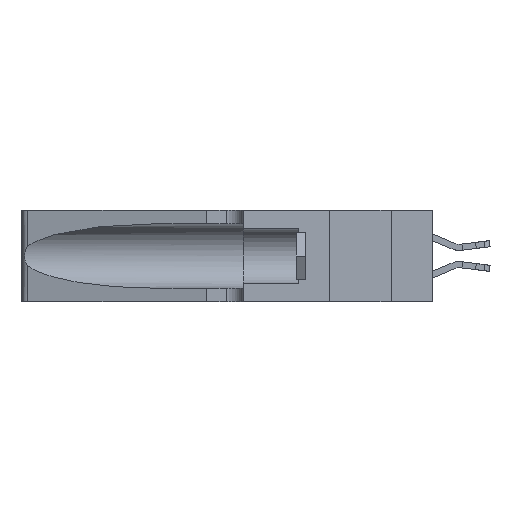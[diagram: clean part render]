
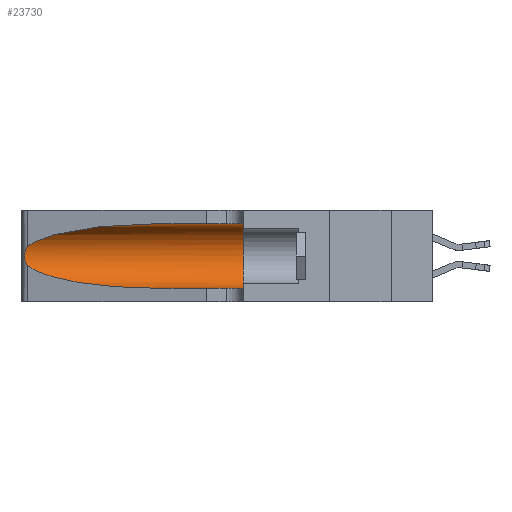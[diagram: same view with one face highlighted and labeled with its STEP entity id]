
A CAD part, left-side view. The second image highlights one B-rep face of the part: STEP entity #23730.
In plain terms, the highlighted cylindrical face has radius 3.308 mm (diameter 6.617 mm), a partial arc.
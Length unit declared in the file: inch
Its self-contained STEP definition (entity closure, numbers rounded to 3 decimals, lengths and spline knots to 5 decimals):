
#177 = DIRECTION ( 'NONE',  ( 0., -1., 0. ) ) ;
#205 = CARTESIAN_POINT ( 'NONE',  ( 0.2373, 1.15595, 0.28018 ) ) ;
#1147 = ORIENTED_EDGE ( 'NONE', *, *, #32298, .T. ) ;
#2047 = CARTESIAN_POINT ( 'NONE',  ( 0.25856, 1.23593, 0.16098 ) ) ;
#2489 = DIRECTION ( 'NONE',  ( 0., -1., 0. ) ) ;
#3336 = ORIENTED_EDGE ( 'NONE', *, *, #33354, .F. ) ;
#4023 = LINE ( 'NONE', #35388, #10461 ) ;
#4152 = DIRECTION ( 'NONE',  ( 0., -1., 0. ) ) ;
#4874 = CARTESIAN_POINT ( 'NONE',  ( 0.25639, 1.23186, 0.15144 ) ) ;
#5517 = CIRCLE ( 'NONE', #25784, 0.13025 ) ;
#5779 = EDGE_CURVE ( 'NONE', #12268, #11957, #31395, .T. ) ;
#5876 = VERTEX_POINT ( 'NONE', #25345 ) ;
#5976 = CARTESIAN_POINT ( 'NONE',  ( 0.1305, 0.72297, 0.05475 ) ) ;
#6512 = EDGE_LOOP ( 'NONE', ( #1147, #16391, #9265, #7586, #3336, #28582 ) ) ;
#6934 = CARTESIAN_POINT ( 'NONE',  ( 0.1305, 1.61858, 0.185 ) ) ;
#7407 = CARTESIAN_POINT ( 'NONE',  ( 0.25487, 1.22718, 0.22369 ) ) ;
#7586 = ORIENTED_EDGE ( 'NONE', *, *, #15427, .T. ) ;
#7638 = CARTESIAN_POINT ( 'NONE',  ( 0.25487, 1.22718, 0.14631 ) ) ;
#8464 = CARTESIAN_POINT ( 'NONE',  ( 0.25487, 1.22718, 0.14631 ) ) ;
#9265 = ORIENTED_EDGE ( 'NONE', *, *, #5779, .T. ) ;
#9838 = VERTEX_POINT ( 'NONE', #24426 ) ;
#10275 = CARTESIAN_POINT ( 'NONE',  ( 0.25639, 1.23184, 0.21858 ) ) ;
#10416 = AXIS2_PLACEMENT_3D ( 'NONE', #6934, #4152, #23348 ) ;
#10423 = DIRECTION ( 'NONE',  ( 0., 1., 0. ) ) ;
#10461 = VECTOR ( 'NONE', #2489, 39.37008 ) ;
#11229 = CARTESIAN_POINT ( 'NONE',  ( 0.18966, 0.96281, 0.31525 ) ) ;
#11402 = CARTESIAN_POINT ( 'NONE',  ( 0.25487, 1.22718, 0.22369 ) ) ;
#11957 = VERTEX_POINT ( 'NONE', #5976 ) ;
#12268 = VERTEX_POINT ( 'NONE', #29209 ) ;
#13074 = CARTESIAN_POINT ( 'NONE',  ( 0.25854, 1.2359, 0.20912 ) ) ;
#13637 = EDGE_CURVE ( 'NONE', #9838, #5876, #19664, .T. ) ;
#15140 = CARTESIAN_POINT ( 'NONE',  ( 0.1305, 0.35, 0.05475 ) ) ;
#15427 = EDGE_CURVE ( 'NONE', #11957, #34701, #4023, .T. ) ;
#15838 = CARTESIAN_POINT ( 'NONE',  ( 0.26075, 1.23896, 0.19203 ) ) ;
#16391 = ORIENTED_EDGE ( 'NONE', *, *, #26355, .T. ) ;
#16588 = VERTEX_POINT ( 'NONE', #11402 ) ;
#18579 = CARTESIAN_POINT ( 'NONE',  ( 0.26017, 1.23833, 0.17102 ) ) ;
#19403 = CARTESIAN_POINT ( 'NONE',  ( 0.18966, 0.96281, 0.05475 ) ) ;
#19521 = CARTESIAN_POINT ( 'NONE',  ( 0.25487, 1.22718, 0.22369 ) ) ;
#19664 = LINE ( 'NONE', #33135, #32472 ) ;
#21328 = CARTESIAN_POINT ( 'NONE',  ( 0.25789, 1.23486, 0.15765 ) ) ;
#22133 = CARTESIAN_POINT ( 'NONE',  ( 0.2373, 1.15595, 0.08982 ) ) ;
#23348 = DIRECTION ( 'NONE',  ( 0., 0., -1. ) ) ;
#23453 =( BOUNDED_CURVE ( )  B_SPLINE_CURVE ( 3, ( #30400, #11229, #205, #19521 ),
 .UNSPECIFIED., .F., .F. ) 
 B_SPLINE_CURVE_WITH_KNOTS ( ( 4, 4 ),
 ( 1.5708, 2.84003 ),
 .UNSPECIFIED. ) 
 CURVE ( )  GEOMETRIC_REPRESENTATION_ITEM ( )  RATIONAL_B_SPLINE_CURVE ( ( 1., 0.87, 0.87, 1. ) ) 
 REPRESENTATION_ITEM ( '' )  );
#23730 = ADVANCED_FACE ( 'NONE', ( #27294 ), #31993, .F. ) ;
#24056 = CARTESIAN_POINT ( 'NONE',  ( 0.25555, 1.22993, 0.14849 ) ) ;
#24426 = CARTESIAN_POINT ( 'NONE',  ( 0.1305, 0.72297, 0.31525 ) ) ;
#25345 = CARTESIAN_POINT ( 'NONE',  ( 0.1305, 0.35, 0.31525 ) ) ;
#25784 = AXIS2_PLACEMENT_3D ( 'NONE', #26841, #10423, #29605 ) ;
#26090 = B_SPLINE_CURVE_WITH_KNOTS ( 'NONE', 3,
 ( #7407, #26691, #10275, #29452, #13074, #32221, #15838, #34953, #18579, #2047, #21328, #4874, #24056, #7638 ),
 .UNSPECIFIED., .F., .F.,
 ( 4, 2, 2, 2, 2, 2, 4 ),
 ( 0., 0.00027, 0.00053, 0.00107, 0.0016, 0.00187, 0.00214 ),
 .UNSPECIFIED. ) ;
#26355 = EDGE_CURVE ( 'NONE', #16588, #12268, #26090, .T. ) ;
#26691 = CARTESIAN_POINT ( 'NONE',  ( 0.25555, 1.22994, 0.2215 ) ) ;
#26841 = CARTESIAN_POINT ( 'NONE',  ( 0.1305, 0.35, 0.185 ) ) ;
#27294 = FACE_OUTER_BOUND ( 'NONE', #6512, .T. ) ;
#27643 = CARTESIAN_POINT ( 'NONE',  ( 0.1305, 0.72297, 0.05475 ) ) ;
#28582 = ORIENTED_EDGE ( 'NONE', *, *, #13637, .F. ) ;
#29209 = CARTESIAN_POINT ( 'NONE',  ( 0.25487, 1.22718, 0.14631 ) ) ;
#29452 = CARTESIAN_POINT ( 'NONE',  ( 0.25787, 1.23484, 0.2124 ) ) ;
#29605 = DIRECTION ( 'NONE',  ( 0., 0., 1. ) ) ;
#30400 = CARTESIAN_POINT ( 'NONE',  ( 0.1305, 0.72297, 0.31525 ) ) ;
#31395 =( BOUNDED_CURVE ( )  B_SPLINE_CURVE ( 3, ( #8464, #22133, #19403, #27643 ),
 .UNSPECIFIED., .F., .F. ) 
 B_SPLINE_CURVE_WITH_KNOTS ( ( 4, 4 ),
 ( 3.44316, 4.71239 ),
 .UNSPECIFIED. ) 
 CURVE ( )  GEOMETRIC_REPRESENTATION_ITEM ( )  RATIONAL_B_SPLINE_CURVE ( ( 1., 0.87, 0.87, 1. ) ) 
 REPRESENTATION_ITEM ( '' )  );
#31993 = CYLINDRICAL_SURFACE ( 'NONE', #10416, 0.13025 ) ;
#32221 = CARTESIAN_POINT ( 'NONE',  ( 0.26018, 1.23835, 0.19895 ) ) ;
#32298 = EDGE_CURVE ( 'NONE', #9838, #16588, #23453, .T. ) ;
#32472 = VECTOR ( 'NONE', #177, 39.37008 ) ;
#33135 = CARTESIAN_POINT ( 'NONE',  ( 0.1305, 1.61858, 0.31525 ) ) ;
#33354 = EDGE_CURVE ( 'NONE', #5876, #34701, #5517, .T. ) ;
#34701 = VERTEX_POINT ( 'NONE', #15140 ) ;
#34953 = CARTESIAN_POINT ( 'NONE',  ( 0.26075, 1.23896, 0.178 ) ) ;
#35388 = CARTESIAN_POINT ( 'NONE',  ( 0.1305, 1.61858, 0.05475 ) ) ;
